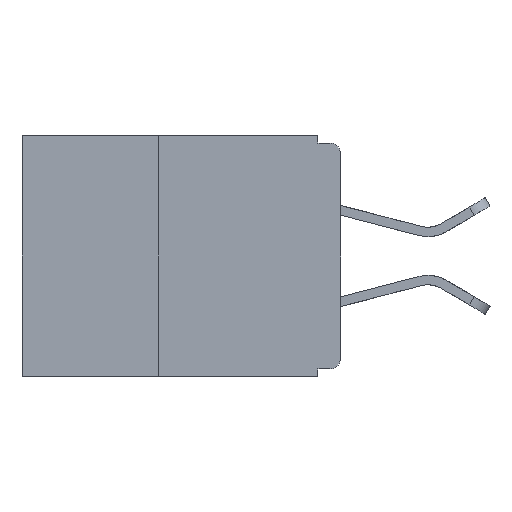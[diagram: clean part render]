
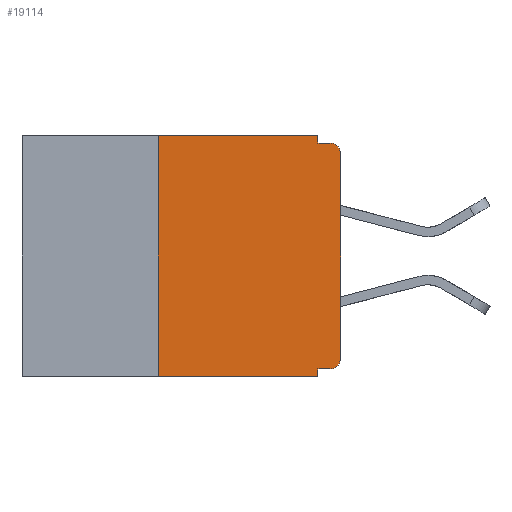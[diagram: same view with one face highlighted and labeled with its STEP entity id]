
A CAD part, left-side view. The second image highlights one B-rep face of the part: STEP entity #19114.
In plain terms, the highlighted planar face has unit normal (-1, 0, 0).
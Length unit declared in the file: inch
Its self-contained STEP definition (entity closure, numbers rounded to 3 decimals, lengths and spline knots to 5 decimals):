
#56 = VECTOR ( 'NONE', #9167, 39.37008 ) ;
#300 = ORIENTED_EDGE ( 'NONE', *, *, #13896, .F. ) ;
#586 = CARTESIAN_POINT ( 'NONE',  ( 0., 0.015, -0.32 ) ) ;
#593 = ORIENTED_EDGE ( 'NONE', *, *, #11448, .F. ) ;
#606 = VECTOR ( 'NONE', #8531, 39.37008 ) ;
#734 = CARTESIAN_POINT ( 'NONE',  ( 0., 0.031, -0.33 ) ) ;
#876 = LINE ( 'NONE', #15365, #4554 ) ;
#1435 = EDGE_CURVE ( 'NONE', #7250, #16108, #876, .T. ) ;
#1530 = EDGE_CURVE ( 'NONE', #12895, #14672, #6729, .T. ) ;
#1750 = EDGE_CURVE ( 'NONE', #10649, #16108, #15235, .T. ) ;
#1771 = LINE ( 'NONE', #12107, #9554 ) ;
#2073 = ORIENTED_EDGE ( 'NONE', *, *, #1530, .T. ) ;
#2425 = CARTESIAN_POINT ( 'NONE',  ( 0., 0.015, -0.01 ) ) ;
#3156 = VECTOR ( 'NONE', #18354, 39.37008 ) ;
#3173 = CARTESIAN_POINT ( 'NONE',  ( 0., 0.031, -0.33 ) ) ;
#3272 = CARTESIAN_POINT ( 'NONE',  ( 0., 0.437, -0.33 ) ) ;
#3507 = ORIENTED_EDGE ( 'NONE', *, *, #1750, .T. ) ;
#3766 = LINE ( 'NONE', #18419, #56 ) ;
#3892 = FACE_OUTER_BOUND ( 'NONE', #18942, .T. ) ;
#4352 = VERTEX_POINT ( 'NONE', #7583 ) ;
#4554 = VECTOR ( 'NONE', #16395, 39.37008 ) ;
#5123 = CARTESIAN_POINT ( 'NONE',  ( 0., 0., -0.305 ) ) ;
#6015 = CARTESIAN_POINT ( 'NONE',  ( 0., 0.25, -0.33 ) ) ;
#6366 = LINE ( 'NONE', #11227, #18254 ) ;
#6449 = CARTESIAN_POINT ( 'NONE',  ( 0., 0., -0.025 ) ) ;
#6598 = AXIS2_PLACEMENT_3D ( 'NONE', #12928, #12884, #8130 ) ;
#6729 = LINE ( 'NONE', #3272, #18605 ) ;
#7150 = VERTEX_POINT ( 'NONE', #586 ) ;
#7250 = VERTEX_POINT ( 'NONE', #17996 ) ;
#7292 = LINE ( 'NONE', #16780, #3156 ) ;
#7583 = CARTESIAN_POINT ( 'NONE',  ( 0., 0.031, 0. ) ) ;
#8130 = DIRECTION ( 'NONE',  ( 0., 0., -1. ) ) ;
#8394 = ORIENTED_EDGE ( 'NONE', *, *, #12879, .F. ) ;
#8531 = DIRECTION ( 'NONE',  ( 0., 0., -1. ) ) ;
#8779 = CARTESIAN_POINT ( 'NONE',  ( 0., 0.031, 0. ) ) ;
#8811 = CIRCLE ( 'NONE', #14737, 0.015 ) ;
#8879 = ORIENTED_EDGE ( 'NONE', *, *, #10223, .F. ) ;
#9053 = DIRECTION ( 'NONE',  ( 0., -1., 0. ) ) ;
#9079 = DIRECTION ( 'NONE',  ( -1., 0., 0. ) ) ;
#9094 = EDGE_CURVE ( 'NONE', #7150, #9352, #8811, .T. ) ;
#9167 = DIRECTION ( 'NONE',  ( 0., 0., 1. ) ) ;
#9352 = VERTEX_POINT ( 'NONE', #5123 ) ;
#9554 = VECTOR ( 'NONE', #9053, 39.37008 ) ;
#9804 = CARTESIAN_POINT ( 'NONE',  ( 0., 0.25, 0. ) ) ;
#10223 = EDGE_CURVE ( 'NONE', #4352, #7250, #19812, .T. ) ;
#10295 = DIRECTION ( 'NONE',  ( 0., 0., -1. ) ) ;
#10419 = PLANE ( 'NONE',  #17037 ) ;
#10649 = VERTEX_POINT ( 'NONE', #6449 ) ;
#11227 = CARTESIAN_POINT ( 'NONE',  ( 0., 0., -0.32 ) ) ;
#11355 = DIRECTION ( 'NONE',  ( 0., -1., 0. ) ) ;
#11448 = EDGE_CURVE ( 'NONE', #14617, #14672, #17162, .T. ) ;
#11522 = DIRECTION ( 'NONE',  ( 0., 0., -1. ) ) ;
#11879 = VERTEX_POINT ( 'NONE', #9804 ) ;
#12107 = CARTESIAN_POINT ( 'NONE',  ( 0., 0.437, 0. ) ) ;
#12595 = ORIENTED_EDGE ( 'NONE', *, *, #9094, .T. ) ;
#12828 = DIRECTION ( 'NONE',  ( 0., 1., 0. ) ) ;
#12879 = EDGE_CURVE ( 'NONE', #12895, #11879, #3766, .T. ) ;
#12884 = DIRECTION ( 'NONE',  ( -1., 0., 0. ) ) ;
#12895 = VERTEX_POINT ( 'NONE', #6015 ) ;
#12928 = CARTESIAN_POINT ( 'NONE',  ( 0., 0.015, -0.025 ) ) ;
#13747 = ORIENTED_EDGE ( 'NONE', *, *, #1435, .F. ) ;
#13896 = EDGE_CURVE ( 'NONE', #11879, #4352, #1771, .T. ) ;
#14617 = VERTEX_POINT ( 'NONE', #18547 ) ;
#14672 = VERTEX_POINT ( 'NONE', #3173 ) ;
#14737 = AXIS2_PLACEMENT_3D ( 'NONE', #18336, #9079, #19824 ) ;
#15199 = DIRECTION ( 'NONE',  ( 1., 0., 0. ) ) ;
#15235 = CIRCLE ( 'NONE', #6598, 0.015 ) ;
#15365 = CARTESIAN_POINT ( 'NONE',  ( 0., 0., -0.01 ) ) ;
#16108 = VERTEX_POINT ( 'NONE', #2425 ) ;
#16239 = VECTOR ( 'NONE', #10295, 39.37008 ) ;
#16395 = DIRECTION ( 'NONE',  ( 0., -1., 0. ) ) ;
#16585 = CARTESIAN_POINT ( 'NONE',  ( 0., 0.437, 0. ) ) ;
#16780 = CARTESIAN_POINT ( 'NONE',  ( 0., 0., 0. ) ) ;
#17037 = AXIS2_PLACEMENT_3D ( 'NONE', #16585, #15199, #11522 ) ;
#17162 = LINE ( 'NONE', #734, #606 ) ;
#17655 = EDGE_CURVE ( 'NONE', #7150, #14617, #6366, .T. ) ;
#17996 = CARTESIAN_POINT ( 'NONE',  ( 0., 0.031, -0.01 ) ) ;
#18254 = VECTOR ( 'NONE', #12828, 39.37008 ) ;
#18336 = CARTESIAN_POINT ( 'NONE',  ( 0., 0.015, -0.305 ) ) ;
#18354 = DIRECTION ( 'NONE',  ( 0., 0., 1. ) ) ;
#18419 = CARTESIAN_POINT ( 'NONE',  ( 0., 0.25, -0.33 ) ) ;
#18547 = CARTESIAN_POINT ( 'NONE',  ( 0., 0.031, -0.32 ) ) ;
#18605 = VECTOR ( 'NONE', #11355, 39.37008 ) ;
#18942 = EDGE_LOOP ( 'NONE', ( #19674, #3507, #13747, #8879, #300, #8394, #2073, #593, #19082, #12595 ) ) ;
#19082 = ORIENTED_EDGE ( 'NONE', *, *, #17655, .F. ) ;
#19114 = ADVANCED_FACE ( 'NONE', ( #3892 ), #10419, .F. ) ;
#19388 = EDGE_CURVE ( 'NONE', #9352, #10649, #7292, .T. ) ;
#19674 = ORIENTED_EDGE ( 'NONE', *, *, #19388, .T. ) ;
#19812 = LINE ( 'NONE', #8779, #16239 ) ;
#19824 = DIRECTION ( 'NONE',  ( 0., 0., -1. ) ) ;
